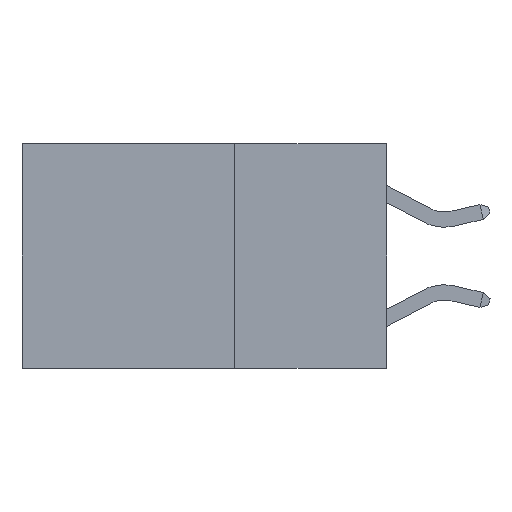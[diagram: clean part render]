
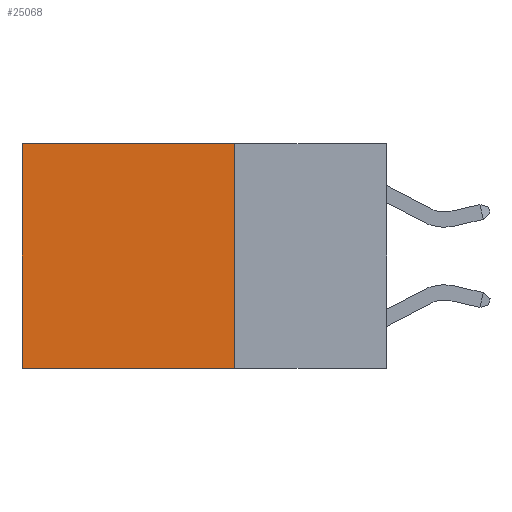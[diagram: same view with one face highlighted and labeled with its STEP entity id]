
A CAD part, left-side view. The second image highlights one B-rep face of the part: STEP entity #25068.
In plain terms, the highlighted planar face has unit normal (-1, 0, 0).
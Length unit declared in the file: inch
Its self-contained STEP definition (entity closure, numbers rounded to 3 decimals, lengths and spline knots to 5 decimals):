
#81 = CARTESIAN_POINT ( 'NONE',  ( 0.2625, 0.25, -0.37 ) ) ;
#678 = VECTOR ( 'NONE', #22423, 39.37008 ) ;
#1169 = VERTEX_POINT ( 'NONE', #12836 ) ;
#2244 = EDGE_LOOP ( 'NONE', ( #21870, #15209, #26015, #6349 ) ) ;
#4599 = VECTOR ( 'NONE', #6805, 39.37008 ) ;
#5994 = CARTESIAN_POINT ( 'NONE',  ( 0.2625, 0.25, 0. ) ) ;
#6146 = PLANE ( 'NONE',  #7998 ) ;
#6349 = ORIENTED_EDGE ( 'NONE', *, *, #11409, .T. ) ;
#6805 = DIRECTION ( 'NONE',  ( 0., 1., 0. ) ) ;
#7998 = AXIS2_PLACEMENT_3D ( 'NONE', #5994, #13402, #20858 ) ;
#8987 = CARTESIAN_POINT ( 'NONE',  ( 0.2625, 0.6, 0. ) ) ;
#9099 = CARTESIAN_POINT ( 'NONE',  ( 0.2625, 0.6, -0.37 ) ) ;
#9506 = EDGE_CURVE ( 'NONE', #1169, #20191, #23758, .T. ) ;
#11409 = EDGE_CURVE ( 'NONE', #1169, #13907, #29042, .T. ) ;
#12176 = CARTESIAN_POINT ( 'NONE',  ( 0.2625, 0.25, 0. ) ) ;
#12317 = CARTESIAN_POINT ( 'NONE',  ( 0.2625, 0.25, -0.37 ) ) ;
#12589 = CARTESIAN_POINT ( 'NONE',  ( 0.2625, 0.6, 0. ) ) ;
#12836 = CARTESIAN_POINT ( 'NONE',  ( 0.2625, 0.25, 0. ) ) ;
#13402 = DIRECTION ( 'NONE',  ( 1., 0., 0. ) ) ;
#13907 = VERTEX_POINT ( 'NONE', #8987 ) ;
#14380 = EDGE_CURVE ( 'NONE', #20191, #18768, #19870, .T. ) ;
#15209 = ORIENTED_EDGE ( 'NONE', *, *, #14380, .F. ) ;
#16214 = VECTOR ( 'NONE', #18941, 39.37008 ) ;
#17439 = LINE ( 'NONE', #12589, #678 ) ;
#18595 = FACE_OUTER_BOUND ( 'NONE', #2244, .T. ) ;
#18768 = VERTEX_POINT ( 'NONE', #9099 ) ;
#18941 = DIRECTION ( 'NONE',  ( 0., 1., 0. ) ) ;
#19357 = EDGE_CURVE ( 'NONE', #13907, #18768, #17439, .T. ) ;
#19870 = LINE ( 'NONE', #81, #4599 ) ;
#20191 = VERTEX_POINT ( 'NONE', #12317 ) ;
#20858 = DIRECTION ( 'NONE',  ( 0., 0., -1. ) ) ;
#21870 = ORIENTED_EDGE ( 'NONE', *, *, #19357, .T. ) ;
#22423 = DIRECTION ( 'NONE',  ( 0., 0., -1. ) ) ;
#23758 = LINE ( 'NONE', #12176, #27098 ) ;
#23882 = CARTESIAN_POINT ( 'NONE',  ( 0.2625, 0.25, 0. ) ) ;
#25068 = ADVANCED_FACE ( 'NONE', ( #18595 ), #6146, .F. ) ;
#26015 = ORIENTED_EDGE ( 'NONE', *, *, #9506, .F. ) ;
#27098 = VECTOR ( 'NONE', #28758, 39.37008 ) ;
#28758 = DIRECTION ( 'NONE',  ( 0., 0., -1. ) ) ;
#29042 = LINE ( 'NONE', #23882, #16214 ) ;
